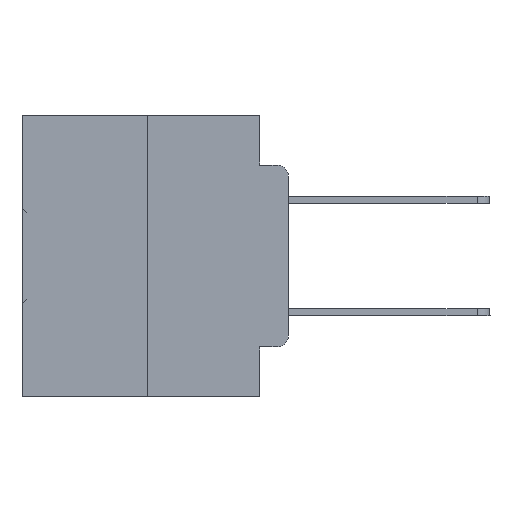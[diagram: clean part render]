
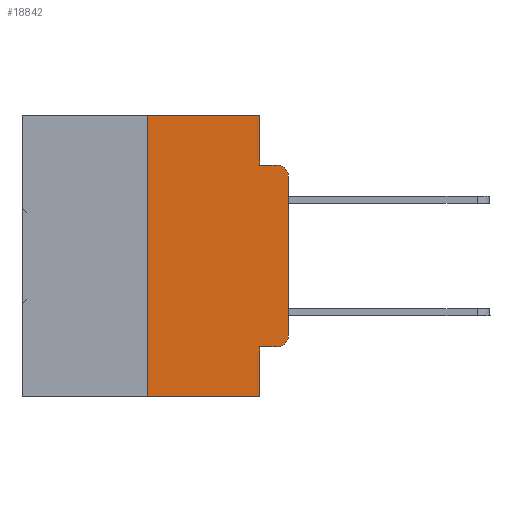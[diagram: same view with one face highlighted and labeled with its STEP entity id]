
A CAD part, left-side view. The second image highlights one B-rep face of the part: STEP entity #18842.
In plain terms, the highlighted planar face has unit normal (-1, 0, 0).
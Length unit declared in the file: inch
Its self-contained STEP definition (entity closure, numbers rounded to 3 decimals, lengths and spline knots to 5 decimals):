
#528 = EDGE_CURVE ( 'NONE', #32745, #15573, #28174, .T. ) ;
#756 = VERTEX_POINT ( 'NONE', #27917 ) ;
#1139 = VERTEX_POINT ( 'NONE', #32352 ) ;
#1274 = DIRECTION ( 'NONE',  ( -1., 0., 0. ) ) ;
#1290 = DIRECTION ( 'NONE',  ( 0., -1., 0. ) ) ;
#1405 = VECTOR ( 'NONE', #17613, 39.37008 ) ;
#1525 = DIRECTION ( 'NONE',  ( 0., 0., -1. ) ) ;
#1665 = VECTOR ( 'NONE', #13563, 39.37008 ) ;
#2028 = EDGE_CURVE ( 'NONE', #1139, #15573, #12571, .T. ) ;
#3614 = EDGE_CURVE ( 'NONE', #756, #25850, #12057, .T. ) ;
#4229 = ORIENTED_EDGE ( 'NONE', *, *, #30009, .F. ) ;
#4571 = CIRCLE ( 'NONE', #5342, 0.02 ) ;
#4791 = DIRECTION ( 'NONE',  ( -1., 0., 0. ) ) ;
#5017 = FACE_OUTER_BOUND ( 'NONE', #9372, .T. ) ;
#5248 = ORIENTED_EDGE ( 'NONE', *, *, #29093, .T. ) ;
#5342 = AXIS2_PLACEMENT_3D ( 'NONE', #15860, #4791, #23812 ) ;
#5699 = DIRECTION ( 'NONE',  ( 0., 0., -1. ) ) ;
#5925 = DIRECTION ( 'NONE',  ( 0., -1., 0. ) ) ;
#6504 = CARTESIAN_POINT ( 'NONE',  ( 0., 0.051, 0. ) ) ;
#7498 = EDGE_CURVE ( 'NONE', #32745, #29255, #11137, .T. ) ;
#7678 = ORIENTED_EDGE ( 'NONE', *, *, #528, .F. ) ;
#8154 = CARTESIAN_POINT ( 'NONE',  ( 0., 0.473, 0. ) ) ;
#8840 = VECTOR ( 'NONE', #18894, 39.37008 ) ;
#9119 = CARTESIAN_POINT ( 'NONE',  ( 0., 0.02, -0.3915 ) ) ;
#9333 = VERTEX_POINT ( 'NONE', #26419 ) ;
#9372 = EDGE_LOOP ( 'NONE', ( #30041, #33796, #29755, #14071, #4229, #16995, #21290, #7678, #10204, #5248 ) ) ;
#9476 = DIRECTION ( 'NONE',  ( 0., 0., -1. ) ) ;
#10204 = ORIENTED_EDGE ( 'NONE', *, *, #7498, .T. ) ;
#10908 = LINE ( 'NONE', #8154, #8840 ) ;
#11018 = PLANE ( 'NONE',  #14835 ) ;
#11137 = LINE ( 'NONE', #24955, #26633 ) ;
#11146 = EDGE_CURVE ( 'NONE', #25850, #30349, #4571, .T. ) ;
#12057 = LINE ( 'NONE', #17481, #1405 ) ;
#12257 = CARTESIAN_POINT ( 'NONE',  ( 0., 0.473, -0.5 ) ) ;
#12571 = LINE ( 'NONE', #12257, #16412 ) ;
#12715 = CIRCLE ( 'NONE', #24705, 0.02 ) ;
#12820 = CARTESIAN_POINT ( 'NONE',  ( 0., 0.25, 0. ) ) ;
#13563 = DIRECTION ( 'NONE',  ( 0., -1., 0. ) ) ;
#13917 = CARTESIAN_POINT ( 'NONE',  ( 0., 0.051, 0. ) ) ;
#14071 = ORIENTED_EDGE ( 'NONE', *, *, #33840, .F. ) ;
#14374 = CARTESIAN_POINT ( 'NONE',  ( 0., 0.051, -0.0885 ) ) ;
#14560 = CARTESIAN_POINT ( 'NONE',  ( 0., 0., -0.1085 ) ) ;
#14835 = AXIS2_PLACEMENT_3D ( 'NONE', #32996, #22058, #5699 ) ;
#15573 = VERTEX_POINT ( 'NONE', #17929 ) ;
#15749 = VECTOR ( 'NONE', #26266, 39.37008 ) ;
#15860 = CARTESIAN_POINT ( 'NONE',  ( 0., 0.02, -0.1085 ) ) ;
#16382 = CARTESIAN_POINT ( 'NONE',  ( 0., 0.25, 0. ) ) ;
#16412 = VECTOR ( 'NONE', #1290, 39.37008 ) ;
#16995 = ORIENTED_EDGE ( 'NONE', *, *, #18238, .F. ) ;
#17481 = CARTESIAN_POINT ( 'NONE',  ( 0., 0., 0. ) ) ;
#17613 = DIRECTION ( 'NONE',  ( 0., 0., 1. ) ) ;
#17929 = CARTESIAN_POINT ( 'NONE',  ( 0., 0.051, -0.5 ) ) ;
#18238 = EDGE_CURVE ( 'NONE', #1139, #21188, #20003, .T. ) ;
#18842 = ADVANCED_FACE ( 'NONE', ( #5017 ), #11018, .F. ) ;
#18894 = DIRECTION ( 'NONE',  ( 0., -1., 0. ) ) ;
#20003 = LINE ( 'NONE', #12820, #15749 ) ;
#20404 = CARTESIAN_POINT ( 'NONE',  ( 0., 0.02, -0.4115 ) ) ;
#21188 = VERTEX_POINT ( 'NONE', #16382 ) ;
#21290 = ORIENTED_EDGE ( 'NONE', *, *, #2028, .T. ) ;
#21634 = CARTESIAN_POINT ( 'NONE',  ( 0., 0.02, -0.0885 ) ) ;
#22058 = DIRECTION ( 'NONE',  ( 1., 0., 0. ) ) ;
#23632 = DIRECTION ( 'NONE',  ( 0., 0., -1. ) ) ;
#23812 = DIRECTION ( 'NONE',  ( 0., 0., -1. ) ) ;
#24705 = AXIS2_PLACEMENT_3D ( 'NONE', #9119, #1274, #9476 ) ;
#24709 = VECTOR ( 'NONE', #23632, 39.37008 ) ;
#24955 = CARTESIAN_POINT ( 'NONE',  ( 0., 0.051, -0.4115 ) ) ;
#25633 = VECTOR ( 'NONE', #1525, 39.37008 ) ;
#25850 = VERTEX_POINT ( 'NONE', #14560 ) ;
#26266 = DIRECTION ( 'NONE',  ( 0., 0., 1. ) ) ;
#26419 = CARTESIAN_POINT ( 'NONE',  ( 0., 0.051, -0.0885 ) ) ;
#26633 = VECTOR ( 'NONE', #5925, 39.37008 ) ;
#27917 = CARTESIAN_POINT ( 'NONE',  ( 0., 0., -0.3915 ) ) ;
#28174 = LINE ( 'NONE', #34909, #24709 ) ;
#28241 = LINE ( 'NONE', #6504, #25633 ) ;
#29030 = EDGE_CURVE ( 'NONE', #9333, #30349, #29790, .T. ) ;
#29093 = EDGE_CURVE ( 'NONE', #29255, #756, #12715, .T. ) ;
#29255 = VERTEX_POINT ( 'NONE', #20404 ) ;
#29263 = CARTESIAN_POINT ( 'NONE',  ( 0., 0.051, -0.4115 ) ) ;
#29755 = ORIENTED_EDGE ( 'NONE', *, *, #29030, .F. ) ;
#29790 = LINE ( 'NONE', #14374, #1665 ) ;
#30009 = EDGE_CURVE ( 'NONE', #21188, #31989, #10908, .T. ) ;
#30041 = ORIENTED_EDGE ( 'NONE', *, *, #3614, .T. ) ;
#30349 = VERTEX_POINT ( 'NONE', #21634 ) ;
#31989 = VERTEX_POINT ( 'NONE', #13917 ) ;
#32352 = CARTESIAN_POINT ( 'NONE',  ( 0., 0.25, -0.5 ) ) ;
#32745 = VERTEX_POINT ( 'NONE', #29263 ) ;
#32996 = CARTESIAN_POINT ( 'NONE',  ( 0., 0.473, 0. ) ) ;
#33796 = ORIENTED_EDGE ( 'NONE', *, *, #11146, .T. ) ;
#33840 = EDGE_CURVE ( 'NONE', #31989, #9333, #28241, .T. ) ;
#34909 = CARTESIAN_POINT ( 'NONE',  ( 0., 0.051, 0. ) ) ;
